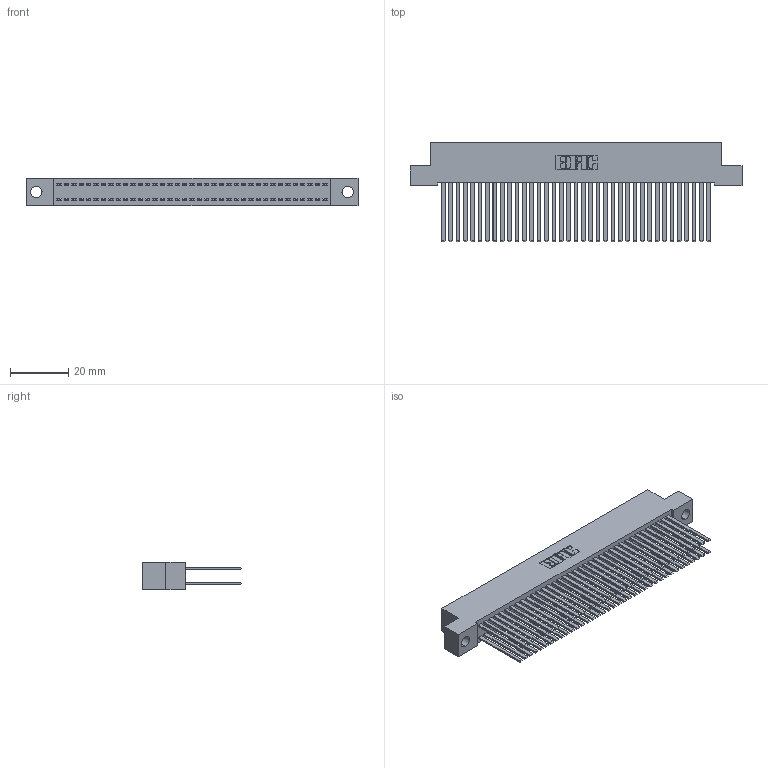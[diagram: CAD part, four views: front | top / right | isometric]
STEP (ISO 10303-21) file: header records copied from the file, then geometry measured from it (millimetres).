
FILE_DESCRIPTION (( 'STEP AP203' ), '1' );
FILE_NAME ('342-074-544-204.STEP', '2019-10-03T17:20:54', ( '' ), ( '' ), 'SwSTEP 2.0', 'SolidWorks 2016', '' );
FILE_SCHEMA (( 'CONFIG_CONTROL_DESIGN' ));
Length unit declared in the file: inch
Products named in the file (3): 345-292-001_345-293-144; 342-074-544-204; 342 Part_.156 TH
Assembly tree (75 placements, depth 2):
  342-074-544-204
    342 Part_.156 TH
    345-292-001_345-293-144  x74
Bounding box: 114.3 x 34.3 x 9.4 mm (x, y, z)
Volume: 11196.5 mm3; surface area: 20798.8 mm2
Topology: 75 solids, 75 shells, 3514 faces, 10437 edges, 6858 vertices
Faces by surface type: plane 2434, cylinder 1080
Entity records: 24137 total; most frequent: CARTESIAN_POINT 4002, ORIENTED_EDGE 3938, DIRECTION 3425, EDGE_CURVE 1969, LINE 1845, VECTOR 1845, VERTEX_POINT 1310, AXIS2_PLACEMENT_3D 790
